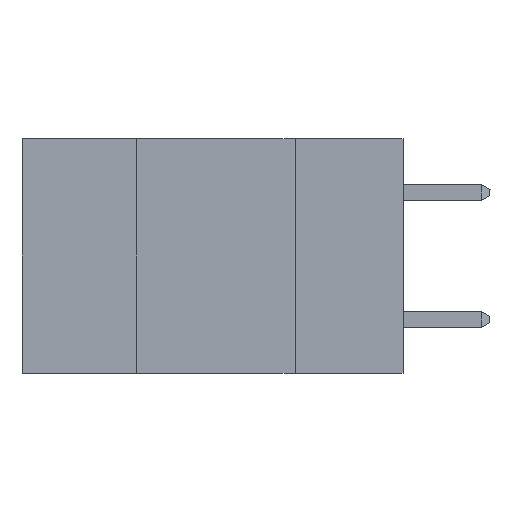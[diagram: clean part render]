
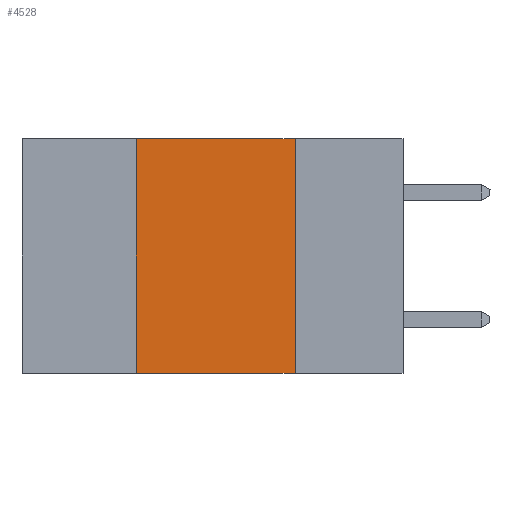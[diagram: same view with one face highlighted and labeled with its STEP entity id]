
A CAD part, left-side view. The second image highlights one B-rep face of the part: STEP entity #4528.
In plain terms, the highlighted planar face has unit normal (-1, 0, 0).
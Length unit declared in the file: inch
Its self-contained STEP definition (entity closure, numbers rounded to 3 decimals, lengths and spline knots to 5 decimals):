
#300 = PLANE ( 'NONE',  #10665 ) ;
#585 = LINE ( 'NONE', #3828, #11536 ) ;
#881 = CARTESIAN_POINT ( 'NONE',  ( 0., 0.17, 0. ) ) ;
#1409 = VECTOR ( 'NONE', #8449, 39.37008 ) ;
#2327 = ORIENTED_EDGE ( 'NONE', *, *, #8209, .F. ) ;
#2430 = VERTEX_POINT ( 'NONE', #4159 ) ;
#2772 = EDGE_CURVE ( 'NONE', #7201, #10812, #3438, .T. ) ;
#3040 = DIRECTION ( 'NONE',  ( 0., -1., 0. ) ) ;
#3438 = LINE ( 'NONE', #11782, #6001 ) ;
#3828 = CARTESIAN_POINT ( 'NONE',  ( 0., 0.42, 0. ) ) ;
#4159 = CARTESIAN_POINT ( 'NONE',  ( 0., 0.17, -0.37 ) ) ;
#4365 = LINE ( 'NONE', #881, #1409 ) ;
#4425 = VERTEX_POINT ( 'NONE', #5071 ) ;
#4528 = ADVANCED_FACE ( 'NONE', ( #12638 ), #300, .F. ) ;
#5071 = CARTESIAN_POINT ( 'NONE',  ( 0., 0.42, -0.37 ) ) ;
#5072 = VECTOR ( 'NONE', #3040, 39.37008 ) ;
#6001 = VECTOR ( 'NONE', #8411, 39.37008 ) ;
#7201 = VERTEX_POINT ( 'NONE', #10816 ) ;
#7207 = CARTESIAN_POINT ( 'NONE',  ( 0., 0.17, 0. ) ) ;
#7810 = DIRECTION ( 'NONE',  ( 0., 0., -1. ) ) ;
#8209 = EDGE_CURVE ( 'NONE', #4425, #7201, #585, .T. ) ;
#8378 = CARTESIAN_POINT ( 'NONE',  ( 0., 0.6, -0.37 ) ) ;
#8386 = ORIENTED_EDGE ( 'NONE', *, *, #2772, .F. ) ;
#8411 = DIRECTION ( 'NONE',  ( 0., -1., 0. ) ) ;
#8449 = DIRECTION ( 'NONE',  ( 0., 0., -1. ) ) ;
#9018 = ORIENTED_EDGE ( 'NONE', *, *, #9589, .T. ) ;
#9144 = CARTESIAN_POINT ( 'NONE',  ( 0., 0.6, 0. ) ) ;
#9163 = EDGE_LOOP ( 'NONE', ( #13410, #8386, #2327, #9018 ) ) ;
#9589 = EDGE_CURVE ( 'NONE', #4425, #2430, #12869, .T. ) ;
#10293 = EDGE_CURVE ( 'NONE', #10812, #2430, #4365, .T. ) ;
#10665 = AXIS2_PLACEMENT_3D ( 'NONE', #9144, #13567, #7810 ) ;
#10812 = VERTEX_POINT ( 'NONE', #7207 ) ;
#10816 = CARTESIAN_POINT ( 'NONE',  ( 0., 0.42, 0. ) ) ;
#11536 = VECTOR ( 'NONE', #13138, 39.37008 ) ;
#11782 = CARTESIAN_POINT ( 'NONE',  ( 0., 0.6, 0. ) ) ;
#12638 = FACE_OUTER_BOUND ( 'NONE', #9163, .T. ) ;
#12869 = LINE ( 'NONE', #8378, #5072 ) ;
#13138 = DIRECTION ( 'NONE',  ( 0., 0., 1. ) ) ;
#13410 = ORIENTED_EDGE ( 'NONE', *, *, #10293, .F. ) ;
#13567 = DIRECTION ( 'NONE',  ( 1., 0., 0. ) ) ;
